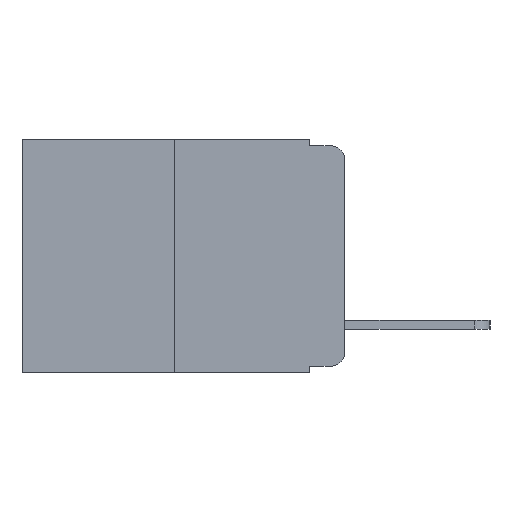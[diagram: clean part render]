
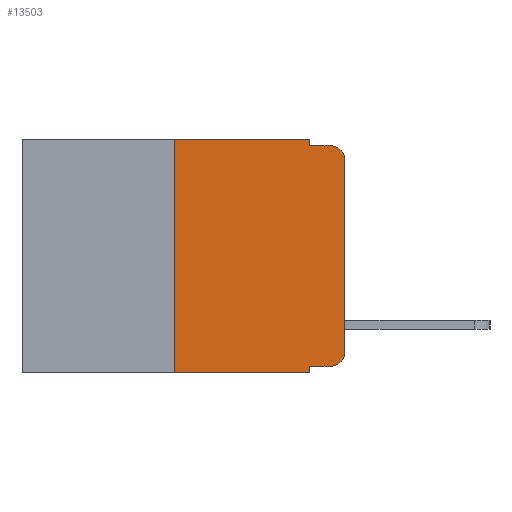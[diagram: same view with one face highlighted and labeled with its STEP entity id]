
A CAD part, left-side view. The second image highlights one B-rep face of the part: STEP entity #13503.
In plain terms, the highlighted planar face has unit normal (-1, 0, 0).
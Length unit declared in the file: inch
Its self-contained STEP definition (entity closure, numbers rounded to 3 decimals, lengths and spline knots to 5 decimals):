
#6 = DIRECTION ( 'NONE',  ( 0., 0., 1. ) ) ;
#188 = CARTESIAN_POINT ( 'NONE',  ( 0., 0.25, 0. ) ) ;
#548 = CARTESIAN_POINT ( 'NONE',  ( 0., 0.25, 0. ) ) ;
#637 = ORIENTED_EDGE ( 'NONE', *, *, #16286, .F. ) ;
#694 = EDGE_CURVE ( 'NONE', #1228, #7434, #16214, .T. ) ;
#1126 = CARTESIAN_POINT ( 'NONE',  ( 0., 0., 0. ) ) ;
#1228 = VERTEX_POINT ( 'NONE', #7409 ) ;
#1288 = ORIENTED_EDGE ( 'NONE', *, *, #6094, .F. ) ;
#1330 = CARTESIAN_POINT ( 'NONE',  ( 0., 0.473, -0.343 ) ) ;
#1452 = LINE ( 'NONE', #1330, #5210 ) ;
#1579 = DIRECTION ( 'NONE',  ( 0., 0., -1. ) ) ;
#1645 = DIRECTION ( 'NONE',  ( 1., 0., 0. ) ) ;
#1717 = CARTESIAN_POINT ( 'NONE',  ( 0., 0.473, 0. ) ) ;
#1744 = PLANE ( 'NONE',  #9948 ) ;
#2912 = EDGE_CURVE ( 'NONE', #8490, #1228, #11582, .T. ) ;
#2947 = DIRECTION ( 'NONE',  ( 0., 0., 1. ) ) ;
#3022 = EDGE_LOOP ( 'NONE', ( #5398, #3646, #637, #11587, #1288, #13300, #9194, #17121, #17777, #8276 ) ) ;
#3149 = DIRECTION ( 'NONE',  ( -1., 0., 0. ) ) ;
#3646 = ORIENTED_EDGE ( 'NONE', *, *, #694, .T. ) ;
#3701 = CARTESIAN_POINT ( 'NONE',  ( 0., 0.02, -0.03 ) ) ;
#3796 = LINE ( 'NONE', #188, #11110 ) ;
#4119 = CARTESIAN_POINT ( 'NONE',  ( 0., 0.051, -0.343 ) ) ;
#4410 = EDGE_CURVE ( 'NONE', #5410, #8490, #18080, .T. ) ;
#4871 = DIRECTION ( 'NONE',  ( 0., 0., -1. ) ) ;
#5210 = VECTOR ( 'NONE', #10457, 39.37008 ) ;
#5398 = ORIENTED_EDGE ( 'NONE', *, *, #2912, .T. ) ;
#5410 = VERTEX_POINT ( 'NONE', #13802 ) ;
#6094 = EDGE_CURVE ( 'NONE', #9014, #6877, #11984, .T. ) ;
#6322 = VERTEX_POINT ( 'NONE', #11804 ) ;
#6408 = EDGE_CURVE ( 'NONE', #10927, #5410, #6732, .T. ) ;
#6468 = VECTOR ( 'NONE', #16114, 39.37008 ) ;
#6497 = CARTESIAN_POINT ( 'NONE',  ( 0., 0.02, -0.01 ) ) ;
#6732 = LINE ( 'NONE', #15181, #10566 ) ;
#6877 = VERTEX_POINT ( 'NONE', #16218 ) ;
#7409 = CARTESIAN_POINT ( 'NONE',  ( 0., 0., -0.03 ) ) ;
#7434 = VERTEX_POINT ( 'NONE', #6497 ) ;
#7551 = LINE ( 'NONE', #10173, #17535 ) ;
#7626 = VERTEX_POINT ( 'NONE', #4119 ) ;
#7748 = VECTOR ( 'NONE', #9241, 39.37008 ) ;
#8008 = VERTEX_POINT ( 'NONE', #14958 ) ;
#8276 = ORIENTED_EDGE ( 'NONE', *, *, #4410, .T. ) ;
#8490 = VERTEX_POINT ( 'NONE', #14445 ) ;
#8810 = VECTOR ( 'NONE', #2947, 39.37008 ) ;
#9014 = VERTEX_POINT ( 'NONE', #548 ) ;
#9194 = ORIENTED_EDGE ( 'NONE', *, *, #16186, .T. ) ;
#9241 = DIRECTION ( 'NONE',  ( 0., -1., 0. ) ) ;
#9948 = AXIS2_PLACEMENT_3D ( 'NONE', #1717, #1645, #1579 ) ;
#10142 = DIRECTION ( 'NONE',  ( 0., 0., -1. ) ) ;
#10173 = CARTESIAN_POINT ( 'NONE',  ( 0., 0.051, 0. ) ) ;
#10289 = EDGE_CURVE ( 'NONE', #10927, #7626, #7551, .T. ) ;
#10457 = DIRECTION ( 'NONE',  ( 0., -1., 0. ) ) ;
#10566 = VECTOR ( 'NONE', #14843, 39.37008 ) ;
#10927 = VERTEX_POINT ( 'NONE', #12961 ) ;
#11060 = CARTESIAN_POINT ( 'NONE',  ( 0., 0.051, 0. ) ) ;
#11110 = VECTOR ( 'NONE', #6, 39.37008 ) ;
#11183 = EDGE_CURVE ( 'NONE', #6322, #9014, #3796, .T. ) ;
#11452 = LINE ( 'NONE', #18056, #7748 ) ;
#11582 = LINE ( 'NONE', #1126, #8810 ) ;
#11587 = ORIENTED_EDGE ( 'NONE', *, *, #15434, .F. ) ;
#11804 = CARTESIAN_POINT ( 'NONE',  ( 0., 0.25, -0.343 ) ) ;
#11951 = LINE ( 'NONE', #11060, #6468 ) ;
#11984 = LINE ( 'NONE', #17196, #14965 ) ;
#12961 = CARTESIAN_POINT ( 'NONE',  ( 0., 0.051, -0.333 ) ) ;
#13300 = ORIENTED_EDGE ( 'NONE', *, *, #11183, .F. ) ;
#13503 = ADVANCED_FACE ( 'NONE', ( #15005 ), #1744, .F. ) ;
#13802 = CARTESIAN_POINT ( 'NONE',  ( 0., 0.02, -0.333 ) ) ;
#14445 = CARTESIAN_POINT ( 'NONE',  ( 0., 0., -0.313 ) ) ;
#14843 = DIRECTION ( 'NONE',  ( 0., -1., 0. ) ) ;
#14958 = CARTESIAN_POINT ( 'NONE',  ( 0., 0.051, -0.01 ) ) ;
#14965 = VECTOR ( 'NONE', #16960, 39.37008 ) ;
#15005 = FACE_OUTER_BOUND ( 'NONE', #3022, .T. ) ;
#15181 = CARTESIAN_POINT ( 'NONE',  ( 0., 0.051, -0.333 ) ) ;
#15434 = EDGE_CURVE ( 'NONE', #6877, #8008, #11951, .T. ) ;
#15913 = DIRECTION ( 'NONE',  ( -1., 0., 0. ) ) ;
#16114 = DIRECTION ( 'NONE',  ( 0., 0., -1. ) ) ;
#16186 = EDGE_CURVE ( 'NONE', #6322, #7626, #1452, .T. ) ;
#16214 = CIRCLE ( 'NONE', #16571, 0.02 ) ;
#16218 = CARTESIAN_POINT ( 'NONE',  ( 0., 0.051, 0. ) ) ;
#16286 = EDGE_CURVE ( 'NONE', #8008, #7434, #11452, .T. ) ;
#16571 = AXIS2_PLACEMENT_3D ( 'NONE', #3701, #3149, #17673 ) ;
#16777 = CARTESIAN_POINT ( 'NONE',  ( 0., 0.02, -0.313 ) ) ;
#16960 = DIRECTION ( 'NONE',  ( 0., -1., 0. ) ) ;
#17121 = ORIENTED_EDGE ( 'NONE', *, *, #10289, .F. ) ;
#17196 = CARTESIAN_POINT ( 'NONE',  ( 0., 0.473, 0. ) ) ;
#17535 = VECTOR ( 'NONE', #10142, 39.37008 ) ;
#17673 = DIRECTION ( 'NONE',  ( 0., 0., -1. ) ) ;
#17763 = AXIS2_PLACEMENT_3D ( 'NONE', #16777, #15913, #4871 ) ;
#17777 = ORIENTED_EDGE ( 'NONE', *, *, #6408, .T. ) ;
#18056 = CARTESIAN_POINT ( 'NONE',  ( 0., 0.051, -0.01 ) ) ;
#18080 = CIRCLE ( 'NONE', #17763, 0.02 ) ;
